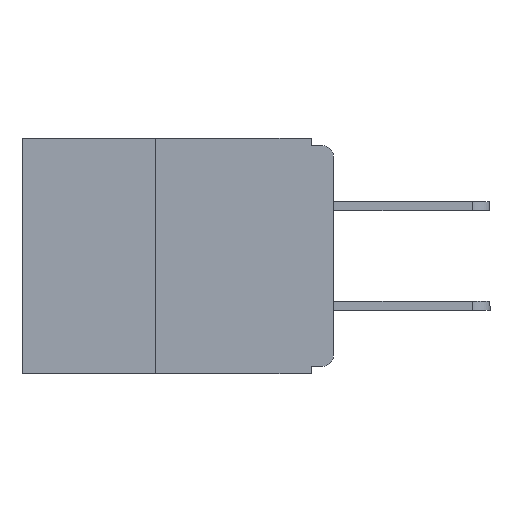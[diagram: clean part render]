
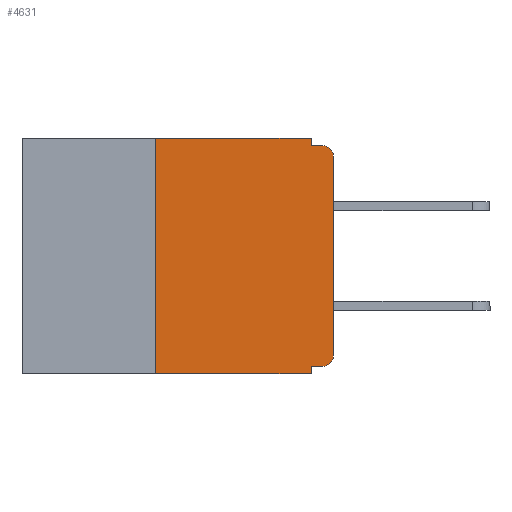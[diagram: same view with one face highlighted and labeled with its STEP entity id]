
A CAD part, left-side view. The second image highlights one B-rep face of the part: STEP entity #4631.
In plain terms, the highlighted planar face has unit normal (-1, 0, 0).
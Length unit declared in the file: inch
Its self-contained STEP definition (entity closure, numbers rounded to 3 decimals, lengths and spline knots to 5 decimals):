
#75 = CARTESIAN_POINT ( 'NONE',  ( 0., 0.031, 0. ) ) ;
#194 = ORIENTED_EDGE ( 'NONE', *, *, #12156, .T. ) ;
#586 = AXIS2_PLACEMENT_3D ( 'NONE', #20886, #20699, #20641 ) ;
#656 = ORIENTED_EDGE ( 'NONE', *, *, #5216, .F. ) ;
#1745 = VERTEX_POINT ( 'NONE', #19534 ) ;
#2124 = CARTESIAN_POINT ( 'NONE',  ( 0., 0., -0.305 ) ) ;
#2132 = DIRECTION ( 'NONE',  ( 0., 0., -1. ) ) ;
#3102 = LINE ( 'NONE', #19178, #19493 ) ;
#3646 = DIRECTION ( 'NONE',  ( 0., 0., 1. ) ) ;
#3893 = CARTESIAN_POINT ( 'NONE',  ( 0., 0., -0.32 ) ) ;
#4141 = VERTEX_POINT ( 'NONE', #2124 ) ;
#4231 = VERTEX_POINT ( 'NONE', #26506 ) ;
#4254 = ORIENTED_EDGE ( 'NONE', *, *, #5606, .F. ) ;
#4296 = EDGE_CURVE ( 'NONE', #22825, #5878, #13318, .T. ) ;
#4333 = DIRECTION ( 'NONE',  ( 0., 1., 0. ) ) ;
#4631 = ADVANCED_FACE ( 'NONE', ( #15987 ), #20735, .F. ) ;
#5216 = EDGE_CURVE ( 'NONE', #4231, #16523, #5279, .T. ) ;
#5279 = LINE ( 'NONE', #11108, #20963 ) ;
#5290 = CARTESIAN_POINT ( 'NONE',  ( 0., 0.437, -0.33 ) ) ;
#5606 = EDGE_CURVE ( 'NONE', #1745, #4231, #9015, .T. ) ;
#5668 = CARTESIAN_POINT ( 'NONE',  ( 0., 0.031, -0.01 ) ) ;
#5878 = VERTEX_POINT ( 'NONE', #75 ) ;
#7447 = DIRECTION ( 'NONE',  ( 0., -1., 0. ) ) ;
#7574 = DIRECTION ( 'NONE',  ( 0., -1., 0. ) ) ;
#7591 = LINE ( 'NONE', #18585, #18921 ) ;
#8481 = DIRECTION ( 'NONE',  ( -1., 0., 0. ) ) ;
#8783 = VECTOR ( 'NONE', #7447, 39.37008 ) ;
#9015 = LINE ( 'NONE', #3893, #9671 ) ;
#9100 = EDGE_CURVE ( 'NONE', #4141, #23043, #3102, .T. ) ;
#9671 = VECTOR ( 'NONE', #4333, 39.37008 ) ;
#9917 = ORIENTED_EDGE ( 'NONE', *, *, #11064, .T. ) ;
#10124 = EDGE_CURVE ( 'NONE', #15645, #26363, #11742, .T. ) ;
#10518 = CIRCLE ( 'NONE', #10834, 0.015 ) ;
#10834 = AXIS2_PLACEMENT_3D ( 'NONE', #21246, #8481, #23360 ) ;
#11015 = DIRECTION ( 'NONE',  ( 0., 0., -1. ) ) ;
#11034 = CARTESIAN_POINT ( 'NONE',  ( 0., 0.031, -0.33 ) ) ;
#11064 = EDGE_CURVE ( 'NONE', #1745, #4141, #26904, .T. ) ;
#11100 = DIRECTION ( 'NONE',  ( 0., 0., -1. ) ) ;
#11108 = CARTESIAN_POINT ( 'NONE',  ( 0., 0.031, -0.33 ) ) ;
#11427 = VECTOR ( 'NONE', #11100, 39.37008 ) ;
#11742 = LINE ( 'NONE', #11850, #22785 ) ;
#11850 = CARTESIAN_POINT ( 'NONE',  ( 0., 0., -0.01 ) ) ;
#12156 = EDGE_CURVE ( 'NONE', #14957, #16523, #25706, .T. ) ;
#12545 = CARTESIAN_POINT ( 'NONE',  ( 0., 0., -0.025 ) ) ;
#13116 = CARTESIAN_POINT ( 'NONE',  ( 0., 0.031, 0. ) ) ;
#13318 = LINE ( 'NONE', #25864, #24651 ) ;
#14925 = DIRECTION ( 'NONE',  ( -1., 0., 0. ) ) ;
#14957 = VERTEX_POINT ( 'NONE', #24572 ) ;
#15209 = AXIS2_PLACEMENT_3D ( 'NONE', #27542, #14925, #2132 ) ;
#15645 = VERTEX_POINT ( 'NONE', #5668 ) ;
#15987 = FACE_OUTER_BOUND ( 'NONE', #23547, .T. ) ;
#16108 = CARTESIAN_POINT ( 'NONE',  ( 0., 0.25, 0. ) ) ;
#16228 = EDGE_CURVE ( 'NONE', #14957, #22825, #7591, .T. ) ;
#16523 = VERTEX_POINT ( 'NONE', #11034 ) ;
#18585 = CARTESIAN_POINT ( 'NONE',  ( 0., 0.25, -0.33 ) ) ;
#18921 = VECTOR ( 'NONE', #3646, 39.37008 ) ;
#19178 = CARTESIAN_POINT ( 'NONE',  ( 0., 0., 0. ) ) ;
#19493 = VECTOR ( 'NONE', #21316, 39.37008 ) ;
#19534 = CARTESIAN_POINT ( 'NONE',  ( 0., 0.015, -0.32 ) ) ;
#19922 = CARTESIAN_POINT ( 'NONE',  ( 0., 0.015, -0.01 ) ) ;
#20641 = DIRECTION ( 'NONE',  ( 0., 0., -1. ) ) ;
#20699 = DIRECTION ( 'NONE',  ( 1., 0., 0. ) ) ;
#20735 = PLANE ( 'NONE',  #586 ) ;
#20886 = CARTESIAN_POINT ( 'NONE',  ( 0., 0.437, 0. ) ) ;
#20963 = VECTOR ( 'NONE', #11015, 39.37008 ) ;
#21246 = CARTESIAN_POINT ( 'NONE',  ( 0., 0.015, -0.025 ) ) ;
#21316 = DIRECTION ( 'NONE',  ( 0., 0., 1. ) ) ;
#21855 = ORIENTED_EDGE ( 'NONE', *, *, #9100, .T. ) ;
#22426 = ORIENTED_EDGE ( 'NONE', *, *, #24537, .T. ) ;
#22670 = ORIENTED_EDGE ( 'NONE', *, *, #10124, .F. ) ;
#22763 = LINE ( 'NONE', #13116, #11427 ) ;
#22785 = VECTOR ( 'NONE', #7574, 39.37008 ) ;
#22825 = VERTEX_POINT ( 'NONE', #16108 ) ;
#22852 = ORIENTED_EDGE ( 'NONE', *, *, #25949, .F. ) ;
#23043 = VERTEX_POINT ( 'NONE', #12545 ) ;
#23360 = DIRECTION ( 'NONE',  ( 0., 0., -1. ) ) ;
#23547 = EDGE_LOOP ( 'NONE', ( #21855, #22426, #22670, #22852, #23688, #26872, #194, #656, #4254, #9917 ) ) ;
#23688 = ORIENTED_EDGE ( 'NONE', *, *, #4296, .F. ) ;
#24537 = EDGE_CURVE ( 'NONE', #23043, #26363, #10518, .T. ) ;
#24572 = CARTESIAN_POINT ( 'NONE',  ( 0., 0.25, -0.33 ) ) ;
#24651 = VECTOR ( 'NONE', #25695, 39.37008 ) ;
#25695 = DIRECTION ( 'NONE',  ( 0., -1., 0. ) ) ;
#25706 = LINE ( 'NONE', #5290, #8783 ) ;
#25864 = CARTESIAN_POINT ( 'NONE',  ( 0., 0.437, 0. ) ) ;
#25949 = EDGE_CURVE ( 'NONE', #5878, #15645, #22763, .T. ) ;
#26363 = VERTEX_POINT ( 'NONE', #19922 ) ;
#26506 = CARTESIAN_POINT ( 'NONE',  ( 0., 0.031, -0.32 ) ) ;
#26872 = ORIENTED_EDGE ( 'NONE', *, *, #16228, .F. ) ;
#26904 = CIRCLE ( 'NONE', #15209, 0.015 ) ;
#27542 = CARTESIAN_POINT ( 'NONE',  ( 0., 0.015, -0.305 ) ) ;
